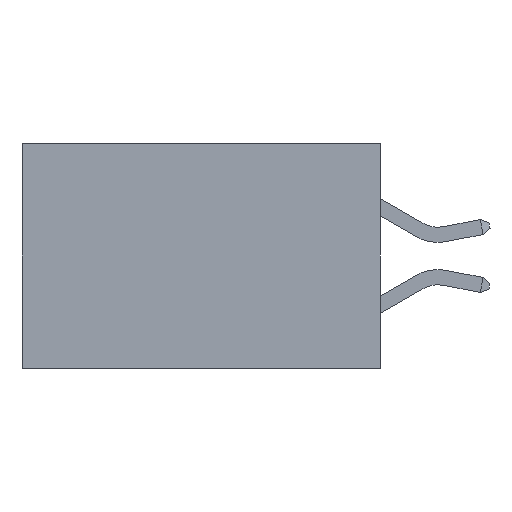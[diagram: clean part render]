
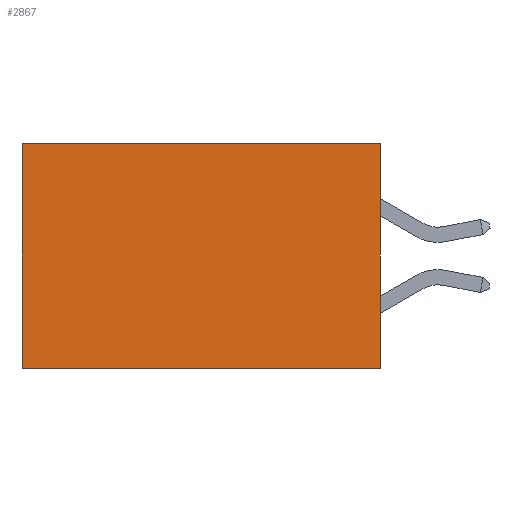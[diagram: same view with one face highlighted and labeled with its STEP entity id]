
A CAD part, left-side view. The second image highlights one B-rep face of the part: STEP entity #2867.
In plain terms, the highlighted planar face has unit normal (-1, 0, 0).
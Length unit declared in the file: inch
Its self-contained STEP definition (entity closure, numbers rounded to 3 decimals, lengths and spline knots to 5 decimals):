
#286 = ORIENTED_EDGE ( 'NONE', *, *, #2182, .T. ) ;
#713 = CARTESIAN_POINT ( 'NONE',  ( 0.277, 0., -0.37 ) ) ;
#989 = EDGE_CURVE ( 'NONE', #6171, #6466, #9311, .T. ) ;
#1126 = VECTOR ( 'NONE', #5261, 39.37008 ) ;
#2182 = EDGE_CURVE ( 'NONE', #6171, #8422, #9628, .T. ) ;
#2277 = ORIENTED_EDGE ( 'NONE', *, *, #989, .F. ) ;
#2600 = VECTOR ( 'NONE', #10137, 39.37008 ) ;
#2836 = EDGE_CURVE ( 'NONE', #6466, #3261, #6327, .T. ) ;
#2867 = ADVANCED_FACE ( 'NONE', ( #7764 ), #5437, .F. ) ;
#3261 = VERTEX_POINT ( 'NONE', #4782 ) ;
#3369 = ORIENTED_EDGE ( 'NONE', *, *, #2836, .F. ) ;
#4782 = CARTESIAN_POINT ( 'NONE',  ( 0.277, 0.59, -0.37 ) ) ;
#4838 = LINE ( 'NONE', #10374, #8696 ) ;
#5090 = ORIENTED_EDGE ( 'NONE', *, *, #9574, .T. ) ;
#5235 = CARTESIAN_POINT ( 'NONE',  ( 0.277, 0., 0. ) ) ;
#5261 = DIRECTION ( 'NONE',  ( 0., 1., 0. ) ) ;
#5295 = DIRECTION ( 'NONE',  ( 0., 0., -1. ) ) ;
#5337 = DIRECTION ( 'NONE',  ( 1., 0., 0. ) ) ;
#5437 = PLANE ( 'NONE',  #8057 ) ;
#6171 = VERTEX_POINT ( 'NONE', #9515 ) ;
#6327 = LINE ( 'NONE', #7161, #10307 ) ;
#6466 = VERTEX_POINT ( 'NONE', #9085 ) ;
#6645 = CARTESIAN_POINT ( 'NONE',  ( 0.277, 0.59, 0. ) ) ;
#6815 = CARTESIAN_POINT ( 'NONE',  ( 0.277, 0., -0.37 ) ) ;
#7161 = CARTESIAN_POINT ( 'NONE',  ( 0.277, 0., -0.37 ) ) ;
#7225 = DIRECTION ( 'NONE',  ( 0., 1., 0. ) ) ;
#7270 = DIRECTION ( 'NONE',  ( 0., 0., -1. ) ) ;
#7764 = FACE_OUTER_BOUND ( 'NONE', #8870, .T. ) ;
#8057 = AXIS2_PLACEMENT_3D ( 'NONE', #6815, #5337, #5295 ) ;
#8422 = VERTEX_POINT ( 'NONE', #6645 ) ;
#8696 = VECTOR ( 'NONE', #7270, 39.37008 ) ;
#8870 = EDGE_LOOP ( 'NONE', ( #5090, #3369, #2277, #286 ) ) ;
#9085 = CARTESIAN_POINT ( 'NONE',  ( 0.277, 0., -0.37 ) ) ;
#9311 = LINE ( 'NONE', #713, #2600 ) ;
#9515 = CARTESIAN_POINT ( 'NONE',  ( 0.277, 0., 0. ) ) ;
#9574 = EDGE_CURVE ( 'NONE', #8422, #3261, #4838, .T. ) ;
#9628 = LINE ( 'NONE', #5235, #1126 ) ;
#10137 = DIRECTION ( 'NONE',  ( 0., 0., -1. ) ) ;
#10307 = VECTOR ( 'NONE', #7225, 39.37008 ) ;
#10374 = CARTESIAN_POINT ( 'NONE',  ( 0.277, 0.59, -0.37 ) ) ;
